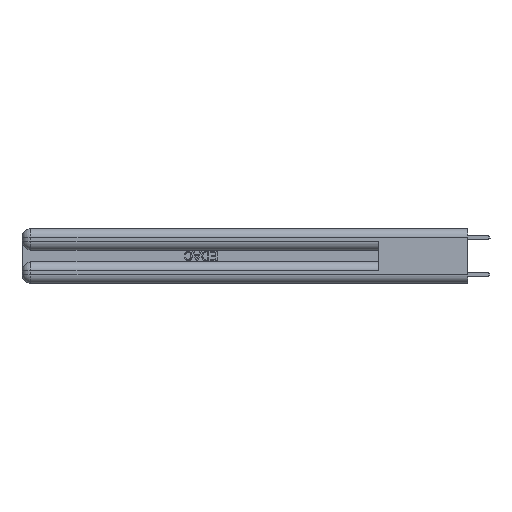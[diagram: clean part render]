
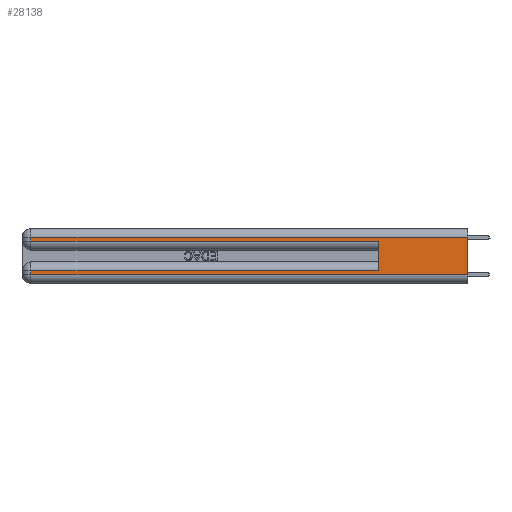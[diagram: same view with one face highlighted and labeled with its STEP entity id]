
A CAD part, left-side view. The second image highlights one B-rep face of the part: STEP entity #28138.
In plain terms, the highlighted planar face has unit normal (-1, 0, 0).
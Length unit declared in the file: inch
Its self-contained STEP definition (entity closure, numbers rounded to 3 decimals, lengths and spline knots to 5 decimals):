
#187 = ORIENTED_EDGE ( 'NONE', *, *, #26782, .F. ) ;
#447 = VERTEX_POINT ( 'NONE', #24115 ) ;
#1041 = VERTEX_POINT ( 'NONE', #13402 ) ;
#1839 = EDGE_CURVE ( 'NONE', #27269, #19695, #4566, .T. ) ;
#2680 = LINE ( 'NONE', #10354, #13708 ) ;
#2802 = EDGE_CURVE ( 'NONE', #19695, #1041, #28873, .T. ) ;
#3616 = CARTESIAN_POINT ( 'NONE',  ( 0., 0.6, 0.085 ) ) ;
#4566 = LINE ( 'NONE', #9824, #20403 ) ;
#4701 = PLANE ( 'NONE',  #23868 ) ;
#4706 = VECTOR ( 'NONE', #33380, 39.37008 ) ;
#4956 = ORIENTED_EDGE ( 'NONE', *, *, #13874, .T. ) ;
#5765 = EDGE_CURVE ( 'NONE', #27269, #16262, #2680, .T. ) ;
#5901 = VECTOR ( 'NONE', #25641, 39.37008 ) ;
#5958 = CARTESIAN_POINT ( 'NONE',  ( 0., 0., 0.31 ) ) ;
#8651 = VECTOR ( 'NONE', #31503, 39.37008 ) ;
#8710 = VERTEX_POINT ( 'NONE', #13610 ) ;
#9230 = VERTEX_POINT ( 'NONE', #11072 ) ;
#9824 = CARTESIAN_POINT ( 'NONE',  ( 0., 0., 0.085 ) ) ;
#10354 = CARTESIAN_POINT ( 'NONE',  ( 0., 0.6, 0.145 ) ) ;
#11072 = CARTESIAN_POINT ( 'NONE',  ( 0., 2.94, 0.285 ) ) ;
#12248 = VECTOR ( 'NONE', #30838, 39.37008 ) ;
#12656 = CARTESIAN_POINT ( 'NONE',  ( 0., 0., 0.37 ) ) ;
#12705 = CARTESIAN_POINT ( 'NONE',  ( 0., 2.94, 0.37 ) ) ;
#12777 = DIRECTION ( 'NONE',  ( 1., 0., 0. ) ) ;
#13157 = LINE ( 'NONE', #23629, #8651 ) ;
#13402 = CARTESIAN_POINT ( 'NONE',  ( 0., 2.94, 0.06 ) ) ;
#13467 = VECTOR ( 'NONE', #33158, 39.37008 ) ;
#13610 = CARTESIAN_POINT ( 'NONE',  ( 0., 0., 0.31 ) ) ;
#13708 = VECTOR ( 'NONE', #31194, 39.37008 ) ;
#13874 = EDGE_CURVE ( 'NONE', #1041, #447, #13157, .T. ) ;
#15905 = LINE ( 'NONE', #22965, #12248 ) ;
#16262 = VERTEX_POINT ( 'NONE', #30768 ) ;
#16360 = LINE ( 'NONE', #5958, #20004 ) ;
#16429 = ORIENTED_EDGE ( 'NONE', *, *, #1839, .T. ) ;
#16561 = VERTEX_POINT ( 'NONE', #24829 ) ;
#17022 = ORIENTED_EDGE ( 'NONE', *, *, #26791, .T. ) ;
#17255 = FACE_OUTER_BOUND ( 'NONE', #25333, .T. ) ;
#18533 = LINE ( 'NONE', #12705, #4706 ) ;
#18994 = EDGE_CURVE ( 'NONE', #9230, #16262, #15905, .T. ) ;
#19695 = VERTEX_POINT ( 'NONE', #27753 ) ;
#20004 = VECTOR ( 'NONE', #23686, 39.37008 ) ;
#20403 = VECTOR ( 'NONE', #22913, 39.37008 ) ;
#20485 = DIRECTION ( 'NONE',  ( 0., 0., -1. ) ) ;
#21225 = ORIENTED_EDGE ( 'NONE', *, *, #2802, .T. ) ;
#21805 = ORIENTED_EDGE ( 'NONE', *, *, #18994, .T. ) ;
#21978 = ORIENTED_EDGE ( 'NONE', *, *, #29466, .T. ) ;
#22913 = DIRECTION ( 'NONE',  ( 0., 1., 0. ) ) ;
#22965 = CARTESIAN_POINT ( 'NONE',  ( 0., 0., 0.285 ) ) ;
#23629 = CARTESIAN_POINT ( 'NONE',  ( 0., 0., 0.06 ) ) ;
#23686 = DIRECTION ( 'NONE',  ( 0., 1., 0. ) ) ;
#23868 = AXIS2_PLACEMENT_3D ( 'NONE', #12656, #12777, #20485 ) ;
#24115 = CARTESIAN_POINT ( 'NONE',  ( 0., 0., 0.06 ) ) ;
#24829 = CARTESIAN_POINT ( 'NONE',  ( 0., 2.94, 0.31 ) ) ;
#25333 = EDGE_LOOP ( 'NONE', ( #187, #21978, #17022, #21805, #27176, #16429, #21225, #4956 ) ) ;
#25641 = DIRECTION ( 'NONE',  ( 0., 0., -1. ) ) ;
#26626 = LINE ( 'NONE', #31010, #5901 ) ;
#26782 = EDGE_CURVE ( 'NONE', #8710, #447, #26626, .T. ) ;
#26791 = EDGE_CURVE ( 'NONE', #16561, #9230, #18533, .T. ) ;
#27176 = ORIENTED_EDGE ( 'NONE', *, *, #5765, .F. ) ;
#27269 = VERTEX_POINT ( 'NONE', #3616 ) ;
#27753 = CARTESIAN_POINT ( 'NONE',  ( 0., 2.94, 0.085 ) ) ;
#27781 = CARTESIAN_POINT ( 'NONE',  ( 0., 2.94, 0.37 ) ) ;
#28138 = ADVANCED_FACE ( 'NONE', ( #17255 ), #4701, .F. ) ;
#28873 = LINE ( 'NONE', #27781, #13467 ) ;
#29466 = EDGE_CURVE ( 'NONE', #8710, #16561, #16360, .T. ) ;
#30768 = CARTESIAN_POINT ( 'NONE',  ( 0., 0.6, 0.285 ) ) ;
#30838 = DIRECTION ( 'NONE',  ( 0., -1., 0. ) ) ;
#31010 = CARTESIAN_POINT ( 'NONE',  ( 0., 0., 0.37 ) ) ;
#31194 = DIRECTION ( 'NONE',  ( 0., 0., 1. ) ) ;
#31503 = DIRECTION ( 'NONE',  ( 0., -1., 0. ) ) ;
#33158 = DIRECTION ( 'NONE',  ( 0., 0., -1. ) ) ;
#33380 = DIRECTION ( 'NONE',  ( 0., 0., -1. ) ) ;
